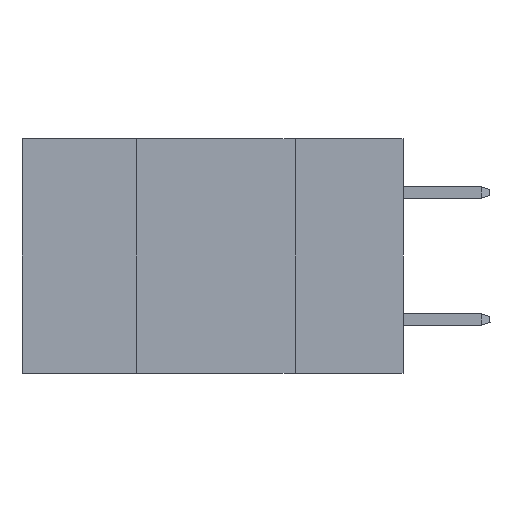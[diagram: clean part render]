
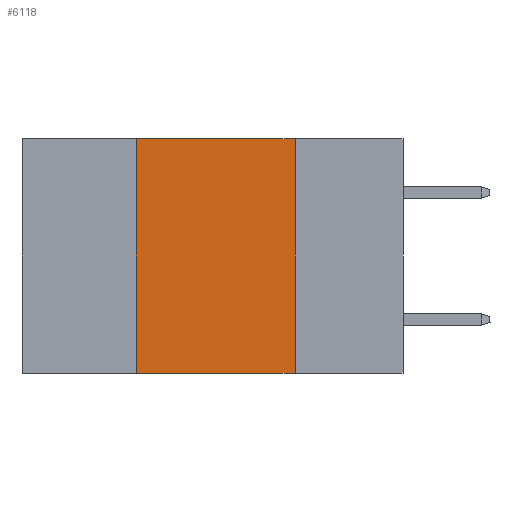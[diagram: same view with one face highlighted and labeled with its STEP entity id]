
A CAD part, left-side view. The second image highlights one B-rep face of the part: STEP entity #6118.
In plain terms, the highlighted planar face has unit normal (-1, 0, 0).
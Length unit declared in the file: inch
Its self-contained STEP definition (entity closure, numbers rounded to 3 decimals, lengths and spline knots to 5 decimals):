
#529 = PLANE ( 'NONE',  #1947 ) ;
#615 = LINE ( 'NONE', #10598, #14290 ) ;
#692 = DIRECTION ( 'NONE',  ( 1., 0., 0. ) ) ;
#1729 = VECTOR ( 'NONE', #14273, 39.37008 ) ;
#1763 = LINE ( 'NONE', #9324, #9012 ) ;
#1857 = CARTESIAN_POINT ( 'NONE',  ( 0., 0.42, -0.37 ) ) ;
#1947 = AXIS2_PLACEMENT_3D ( 'NONE', #10758, #692, #15772 ) ;
#3335 = FACE_OUTER_BOUND ( 'NONE', #12801, .T. ) ;
#3586 = VERTEX_POINT ( 'NONE', #14146 ) ;
#4245 = ORIENTED_EDGE ( 'NONE', *, *, #11521, .T. ) ;
#5264 = VERTEX_POINT ( 'NONE', #14052 ) ;
#6118 = ADVANCED_FACE ( 'NONE', ( #3335 ), #529, .F. ) ;
#6528 = EDGE_CURVE ( 'NONE', #3586, #5264, #9692, .T. ) ;
#7233 = VERTEX_POINT ( 'NONE', #1857 ) ;
#7476 = EDGE_CURVE ( 'NONE', #7233, #15331, #1763, .T. ) ;
#8212 = VECTOR ( 'NONE', #13610, 39.37008 ) ;
#8821 = EDGE_CURVE ( 'NONE', #15331, #3586, #10293, .T. ) ;
#9012 = VECTOR ( 'NONE', #11814, 39.37008 ) ;
#9299 = ORIENTED_EDGE ( 'NONE', *, *, #8821, .F. ) ;
#9324 = CARTESIAN_POINT ( 'NONE',  ( 0., 0.42, 0. ) ) ;
#9692 = LINE ( 'NONE', #14838, #8212 ) ;
#10069 = ORIENTED_EDGE ( 'NONE', *, *, #6528, .F. ) ;
#10293 = LINE ( 'NONE', #10362, #1729 ) ;
#10362 = CARTESIAN_POINT ( 'NONE',  ( 0., 0.6, 0. ) ) ;
#10598 = CARTESIAN_POINT ( 'NONE',  ( 0., 0.6, -0.37 ) ) ;
#10758 = CARTESIAN_POINT ( 'NONE',  ( 0., 0.6, 0. ) ) ;
#10907 = CARTESIAN_POINT ( 'NONE',  ( 0., 0.42, 0. ) ) ;
#11521 = EDGE_CURVE ( 'NONE', #7233, #5264, #615, .T. ) ;
#11814 = DIRECTION ( 'NONE',  ( 0., 0., 1. ) ) ;
#12243 = ORIENTED_EDGE ( 'NONE', *, *, #7476, .F. ) ;
#12801 = EDGE_LOOP ( 'NONE', ( #10069, #9299, #12243, #4245 ) ) ;
#13610 = DIRECTION ( 'NONE',  ( 0., 0., -1. ) ) ;
#14052 = CARTESIAN_POINT ( 'NONE',  ( 0., 0.17, -0.37 ) ) ;
#14146 = CARTESIAN_POINT ( 'NONE',  ( 0., 0.17, 0. ) ) ;
#14273 = DIRECTION ( 'NONE',  ( 0., -1., 0. ) ) ;
#14290 = VECTOR ( 'NONE', #15607, 39.37008 ) ;
#14838 = CARTESIAN_POINT ( 'NONE',  ( 0., 0.17, 0. ) ) ;
#15331 = VERTEX_POINT ( 'NONE', #10907 ) ;
#15607 = DIRECTION ( 'NONE',  ( 0., -1., 0. ) ) ;
#15772 = DIRECTION ( 'NONE',  ( 0., 0., -1. ) ) ;
